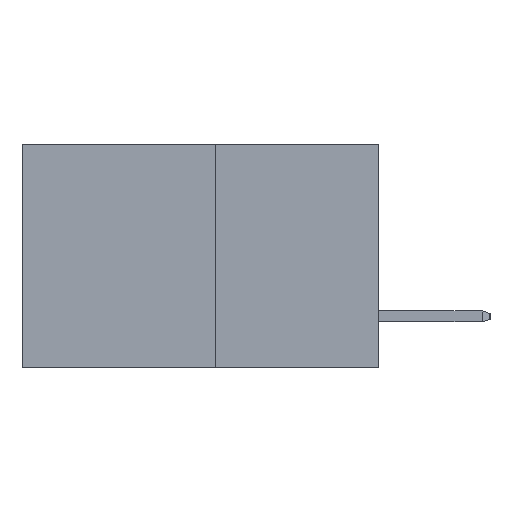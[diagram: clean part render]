
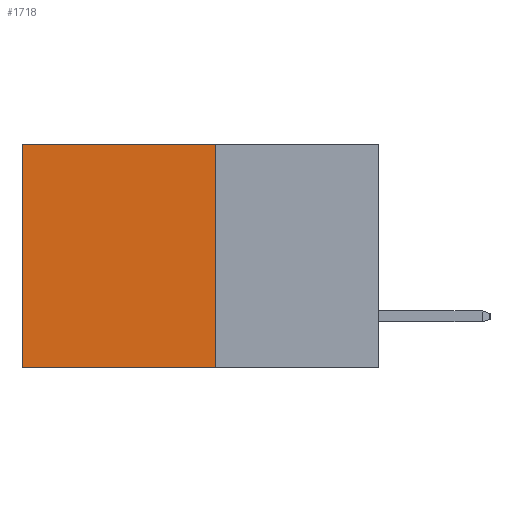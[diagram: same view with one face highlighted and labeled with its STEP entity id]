
A CAD part, left-side view. The second image highlights one B-rep face of the part: STEP entity #1718.
In plain terms, the highlighted planar face has unit normal (-1, 0, 0).
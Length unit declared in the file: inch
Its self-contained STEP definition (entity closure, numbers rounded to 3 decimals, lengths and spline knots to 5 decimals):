
#65 = ORIENTED_EDGE ( 'NONE', *, *, #9485, .F. ) ;
#170 = ORIENTED_EDGE ( 'NONE', *, *, #2268, .T. ) ;
#519 = VERTEX_POINT ( 'NONE', #7153 ) ;
#910 = CARTESIAN_POINT ( 'NONE',  ( 0.277, 0.27, -0.37 ) ) ;
#1071 = CARTESIAN_POINT ( 'NONE',  ( 0.277, 0.59, -0.37 ) ) ;
#1090 = DIRECTION ( 'NONE',  ( 0., 0., -1. ) ) ;
#1718 = ADVANCED_FACE ( 'NONE', ( #5623 ), #6626, .F. ) ;
#1738 = CARTESIAN_POINT ( 'NONE',  ( 0.277, 0.27, 0. ) ) ;
#1806 = VERTEX_POINT ( 'NONE', #3060 ) ;
#1995 = DIRECTION ( 'NONE',  ( 0., 0., -1. ) ) ;
#2234 = LINE ( 'NONE', #910, #9775 ) ;
#2268 = EDGE_CURVE ( 'NONE', #519, #1806, #11984, .T. ) ;
#2393 = LINE ( 'NONE', #8138, #7415 ) ;
#3060 = CARTESIAN_POINT ( 'NONE',  ( 0.277, 0.59, -0.37 ) ) ;
#4199 = ORIENTED_EDGE ( 'NONE', *, *, #8713, .T. ) ;
#5411 = CARTESIAN_POINT ( 'NONE',  ( 0.277, 0.27, 0. ) ) ;
#5623 = FACE_OUTER_BOUND ( 'NONE', #9713, .T. ) ;
#6506 = DIRECTION ( 'NONE',  ( 0., 0., -1. ) ) ;
#6516 = DIRECTION ( 'NONE',  ( 1., 0., 0. ) ) ;
#6626 = PLANE ( 'NONE',  #6852 ) ;
#6743 = EDGE_CURVE ( 'NONE', #11194, #1806, #2393, .T. ) ;
#6852 = AXIS2_PLACEMENT_3D ( 'NONE', #6895, #6516, #6506 ) ;
#6895 = CARTESIAN_POINT ( 'NONE',  ( 0.277, 0.27, -0.37 ) ) ;
#7116 = VERTEX_POINT ( 'NONE', #5411 ) ;
#7153 = CARTESIAN_POINT ( 'NONE',  ( 0.277, 0.59, 0. ) ) ;
#7415 = VECTOR ( 'NONE', #8108, 39.37008 ) ;
#7883 = ORIENTED_EDGE ( 'NONE', *, *, #6743, .F. ) ;
#7932 = CARTESIAN_POINT ( 'NONE',  ( 0.277, 0.27, -0.37 ) ) ;
#8108 = DIRECTION ( 'NONE',  ( 0., 1., 0. ) ) ;
#8138 = CARTESIAN_POINT ( 'NONE',  ( 0.277, 0.27, -0.37 ) ) ;
#8267 = LINE ( 'NONE', #1738, #10718 ) ;
#8713 = EDGE_CURVE ( 'NONE', #7116, #519, #8267, .T. ) ;
#9485 = EDGE_CURVE ( 'NONE', #7116, #11194, #2234, .T. ) ;
#9713 = EDGE_LOOP ( 'NONE', ( #170, #7883, #65, #4199 ) ) ;
#9775 = VECTOR ( 'NONE', #1995, 39.37008 ) ;
#9811 = VECTOR ( 'NONE', #1090, 39.37008 ) ;
#10718 = VECTOR ( 'NONE', #12334, 39.37008 ) ;
#11194 = VERTEX_POINT ( 'NONE', #7932 ) ;
#11984 = LINE ( 'NONE', #1071, #9811 ) ;
#12334 = DIRECTION ( 'NONE',  ( 0., 1., 0. ) ) ;
